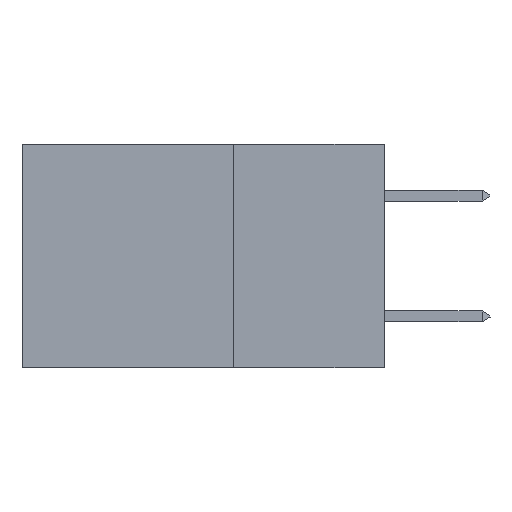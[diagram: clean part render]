
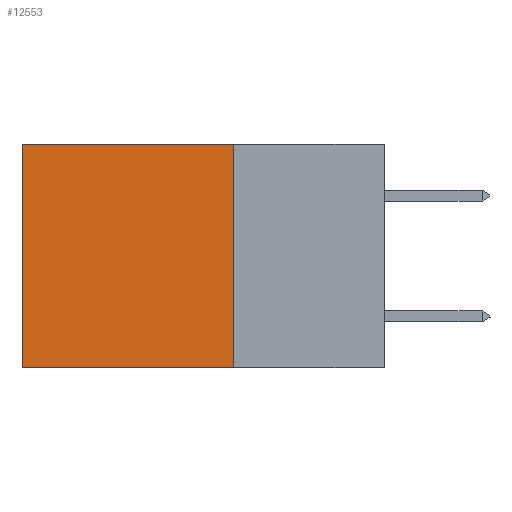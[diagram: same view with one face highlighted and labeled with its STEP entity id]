
A CAD part, left-side view. The second image highlights one B-rep face of the part: STEP entity #12553.
In plain terms, the highlighted planar face has unit normal (-1, 0, 0).
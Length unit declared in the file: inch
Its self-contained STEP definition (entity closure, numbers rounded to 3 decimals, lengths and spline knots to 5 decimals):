
#102 = EDGE_CURVE ( 'NONE', #2357, #11981, #12407, .T. ) ;
#593 = VECTOR ( 'NONE', #9417, 39.37008 ) ;
#809 = VECTOR ( 'NONE', #6744, 39.37008 ) ;
#1540 = FACE_OUTER_BOUND ( 'NONE', #13404, .T. ) ;
#1602 = EDGE_CURVE ( 'NONE', #2808, #7501, #10774, .T. ) ;
#1715 = LINE ( 'NONE', #12560, #809 ) ;
#2086 = DIRECTION ( 'NONE',  ( 0., 1., 0. ) ) ;
#2357 = VERTEX_POINT ( 'NONE', #10223 ) ;
#2412 = CARTESIAN_POINT ( 'NONE',  ( 0.2875, 0.25, 0. ) ) ;
#2808 = VERTEX_POINT ( 'NONE', #12506 ) ;
#2903 = PLANE ( 'NONE',  #8590 ) ;
#2981 = VECTOR ( 'NONE', #3927, 39.37008 ) ;
#3927 = DIRECTION ( 'NONE',  ( 0., 0., -1. ) ) ;
#4426 = ORIENTED_EDGE ( 'NONE', *, *, #102, .T. ) ;
#6092 = CARTESIAN_POINT ( 'NONE',  ( 0.2875, 0.6, -0.37 ) ) ;
#6118 = CARTESIAN_POINT ( 'NONE',  ( 0.2875, 0.25, 0. ) ) ;
#6744 = DIRECTION ( 'NONE',  ( 0., 0., -1. ) ) ;
#6902 = LINE ( 'NONE', #2412, #2981 ) ;
#7034 = ORIENTED_EDGE ( 'NONE', *, *, #1602, .F. ) ;
#7219 = ORIENTED_EDGE ( 'NONE', *, *, #12697, .T. ) ;
#7501 = VERTEX_POINT ( 'NONE', #6092 ) ;
#7736 = ORIENTED_EDGE ( 'NONE', *, *, #12960, .F. ) ;
#8590 = AXIS2_PLACEMENT_3D ( 'NONE', #13165, #9770, #10913 ) ;
#9417 = DIRECTION ( 'NONE',  ( 0., 1., 0. ) ) ;
#9770 = DIRECTION ( 'NONE',  ( 1., 0., 0. ) ) ;
#10223 = CARTESIAN_POINT ( 'NONE',  ( 0.2875, 0.25, 0. ) ) ;
#10774 = LINE ( 'NONE', #12425, #12050 ) ;
#10843 = CARTESIAN_POINT ( 'NONE',  ( 0.2875, 0.6, 0. ) ) ;
#10913 = DIRECTION ( 'NONE',  ( 0., 0., -1. ) ) ;
#11981 = VERTEX_POINT ( 'NONE', #10843 ) ;
#12050 = VECTOR ( 'NONE', #2086, 39.37008 ) ;
#12407 = LINE ( 'NONE', #6118, #593 ) ;
#12425 = CARTESIAN_POINT ( 'NONE',  ( 0.2875, 0.25, -0.37 ) ) ;
#12506 = CARTESIAN_POINT ( 'NONE',  ( 0.2875, 0.25, -0.37 ) ) ;
#12553 = ADVANCED_FACE ( 'NONE', ( #1540 ), #2903, .F. ) ;
#12560 = CARTESIAN_POINT ( 'NONE',  ( 0.2875, 0.6, 0. ) ) ;
#12697 = EDGE_CURVE ( 'NONE', #11981, #7501, #1715, .T. ) ;
#12960 = EDGE_CURVE ( 'NONE', #2357, #2808, #6902, .T. ) ;
#13165 = CARTESIAN_POINT ( 'NONE',  ( 0.2875, 0.25, 0. ) ) ;
#13404 = EDGE_LOOP ( 'NONE', ( #7219, #7034, #7736, #4426 ) ) ;
